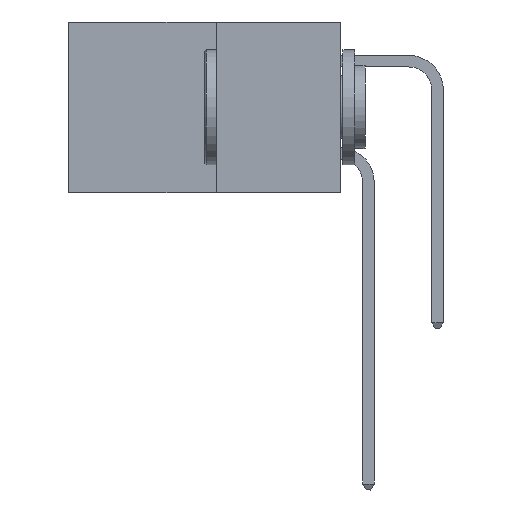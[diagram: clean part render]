
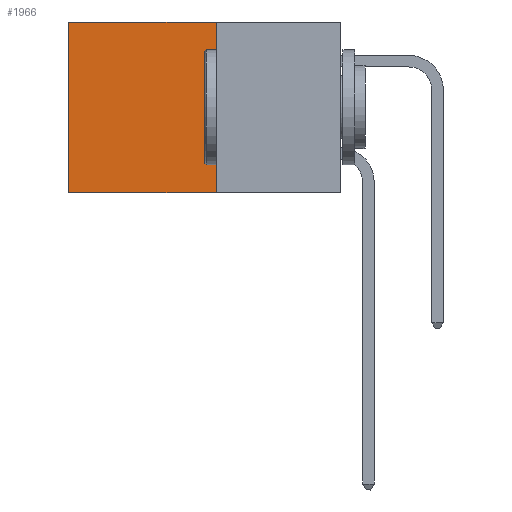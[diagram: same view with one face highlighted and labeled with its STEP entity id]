
A CAD part, left-side view. The second image highlights one B-rep face of the part: STEP entity #1966.
In plain terms, the highlighted planar face has unit normal (-1, 0, 0).
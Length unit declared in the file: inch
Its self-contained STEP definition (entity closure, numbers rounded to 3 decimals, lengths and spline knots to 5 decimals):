
#468 = LINE ( 'NONE', #8154, #3308 ) ;
#674 = AXIS2_PLACEMENT_3D ( 'NONE', #4547, #2580, #1812 ) ;
#1377 = LINE ( 'NONE', #5026, #12410 ) ;
#1812 = DIRECTION ( 'NONE',  ( 0., 0., -1. ) ) ;
#1966 = ADVANCED_FACE ( 'NONE', ( #7395 ), #3586, .F. ) ;
#2127 = ORIENTED_EDGE ( 'NONE', *, *, #3619, .F. ) ;
#2580 = DIRECTION ( 'NONE',  ( 1., 0., 0. ) ) ;
#3308 = VECTOR ( 'NONE', #8141, 39.37008 ) ;
#3586 = PLANE ( 'NONE',  #674 ) ;
#3619 = EDGE_CURVE ( 'NONE', #11418, #7232, #5403, .T. ) ;
#4074 = VERTEX_POINT ( 'NONE', #11977 ) ;
#4308 = ORIENTED_EDGE ( 'NONE', *, *, #7757, .F. ) ;
#4547 = CARTESIAN_POINT ( 'NONE',  ( 0.277, 0.27, -0.37 ) ) ;
#5026 = CARTESIAN_POINT ( 'NONE',  ( 0.277, 0.27, 0. ) ) ;
#5403 = LINE ( 'NONE', #7394, #10559 ) ;
#5847 = LINE ( 'NONE', #6900, #8897 ) ;
#5856 = DIRECTION ( 'NONE',  ( 0., 0., -1. ) ) ;
#6826 = CARTESIAN_POINT ( 'NONE',  ( 0.277, 0.27, -0.37 ) ) ;
#6900 = CARTESIAN_POINT ( 'NONE',  ( 0.277, 0.59, -0.37 ) ) ;
#7232 = VERTEX_POINT ( 'NONE', #6826 ) ;
#7275 = EDGE_LOOP ( 'NONE', ( #9162, #4308, #2127, #10458 ) ) ;
#7319 = VERTEX_POINT ( 'NONE', #11860 ) ;
#7366 = DIRECTION ( 'NONE',  ( 0., 0., -1. ) ) ;
#7394 = CARTESIAN_POINT ( 'NONE',  ( 0.277, 0.27, -0.37 ) ) ;
#7395 = FACE_OUTER_BOUND ( 'NONE', #7275, .T. ) ;
#7757 = EDGE_CURVE ( 'NONE', #7232, #4074, #468, .T. ) ;
#8141 = DIRECTION ( 'NONE',  ( 0., 1., 0. ) ) ;
#8154 = CARTESIAN_POINT ( 'NONE',  ( 0.277, 0.27, -0.37 ) ) ;
#8897 = VECTOR ( 'NONE', #5856, 39.37008 ) ;
#9162 = ORIENTED_EDGE ( 'NONE', *, *, #12155, .T. ) ;
#10152 = DIRECTION ( 'NONE',  ( 0., 1., 0. ) ) ;
#10458 = ORIENTED_EDGE ( 'NONE', *, *, #11004, .T. ) ;
#10559 = VECTOR ( 'NONE', #7366, 39.37008 ) ;
#11004 = EDGE_CURVE ( 'NONE', #11418, #7319, #1377, .T. ) ;
#11418 = VERTEX_POINT ( 'NONE', #11801 ) ;
#11801 = CARTESIAN_POINT ( 'NONE',  ( 0.277, 0.27, 0. ) ) ;
#11860 = CARTESIAN_POINT ( 'NONE',  ( 0.277, 0.59, 0. ) ) ;
#11977 = CARTESIAN_POINT ( 'NONE',  ( 0.277, 0.59, -0.37 ) ) ;
#12155 = EDGE_CURVE ( 'NONE', #7319, #4074, #5847, .T. ) ;
#12410 = VECTOR ( 'NONE', #10152, 39.37008 ) ;
